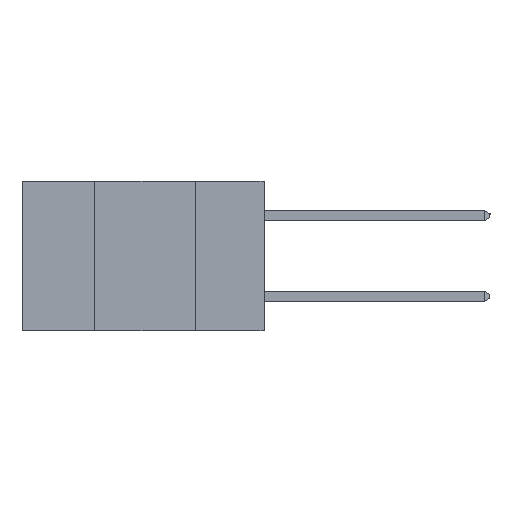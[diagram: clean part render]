
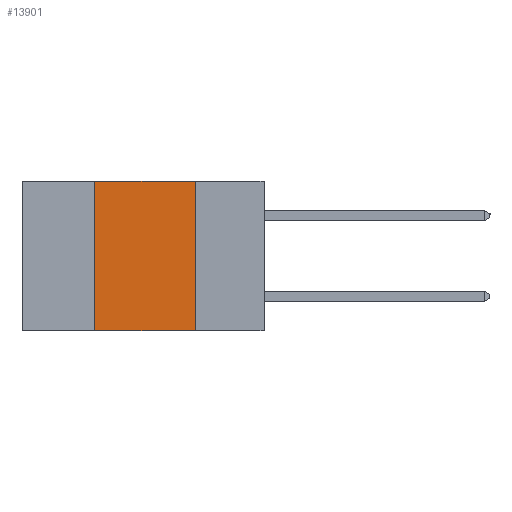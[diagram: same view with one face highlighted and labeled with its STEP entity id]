
A CAD part, left-side view. The second image highlights one B-rep face of the part: STEP entity #13901.
In plain terms, the highlighted planar face has unit normal (-1, 0, 0).
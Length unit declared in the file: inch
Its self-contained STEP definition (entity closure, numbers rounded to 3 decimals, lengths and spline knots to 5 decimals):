
#618 = EDGE_CURVE ( 'NONE', #12036, #2207, #12353, .T. ) ;
#1179 = CARTESIAN_POINT ( 'NONE',  ( 0., 0.6, 0. ) ) ;
#1736 = ORIENTED_EDGE ( 'NONE', *, *, #618, .F. ) ;
#1987 = DIRECTION ( 'NONE',  ( 0., 0., -1. ) ) ;
#2114 = ORIENTED_EDGE ( 'NONE', *, *, #3849, .F. ) ;
#2206 = DIRECTION ( 'NONE',  ( 0., -1., 0. ) ) ;
#2207 = VERTEX_POINT ( 'NONE', #3233 ) ;
#3233 = CARTESIAN_POINT ( 'NONE',  ( 0., 0.17, 0. ) ) ;
#3514 = AXIS2_PLACEMENT_3D ( 'NONE', #7386, #8438, #1987 ) ;
#3680 = VECTOR ( 'NONE', #2206, 39.37008 ) ;
#3693 = ORIENTED_EDGE ( 'NONE', *, *, #11956, .F. ) ;
#3723 = CARTESIAN_POINT ( 'NONE',  ( 0., 0.17, 0. ) ) ;
#3849 = EDGE_CURVE ( 'NONE', #11687, #12036, #4793, .T. ) ;
#4117 = VECTOR ( 'NONE', #4832, 39.37008 ) ;
#4793 = LINE ( 'NONE', #12039, #7367 ) ;
#4832 = DIRECTION ( 'NONE',  ( 0., 0., -1. ) ) ;
#6287 = PLANE ( 'NONE',  #3514 ) ;
#6577 = CARTESIAN_POINT ( 'NONE',  ( 0., 0.42, -0.37 ) ) ;
#6735 = CARTESIAN_POINT ( 'NONE',  ( 0., 0.6, -0.37 ) ) ;
#6781 = DIRECTION ( 'NONE',  ( 0., -1., 0. ) ) ;
#6821 = FACE_OUTER_BOUND ( 'NONE', #9806, .T. ) ;
#7367 = VECTOR ( 'NONE', #11407, 39.37008 ) ;
#7386 = CARTESIAN_POINT ( 'NONE',  ( 0., 0.6, 0. ) ) ;
#8438 = DIRECTION ( 'NONE',  ( 1., 0., 0. ) ) ;
#8745 = LINE ( 'NONE', #6735, #11304 ) ;
#9363 = EDGE_CURVE ( 'NONE', #11687, #9488, #8745, .T. ) ;
#9488 = VERTEX_POINT ( 'NONE', #11767 ) ;
#9806 = EDGE_LOOP ( 'NONE', ( #3693, #1736, #2114, #13989 ) ) ;
#11304 = VECTOR ( 'NONE', #6781, 39.37008 ) ;
#11407 = DIRECTION ( 'NONE',  ( 0., 0., 1. ) ) ;
#11687 = VERTEX_POINT ( 'NONE', #6577 ) ;
#11767 = CARTESIAN_POINT ( 'NONE',  ( 0., 0.17, -0.37 ) ) ;
#11956 = EDGE_CURVE ( 'NONE', #2207, #9488, #13119, .T. ) ;
#12036 = VERTEX_POINT ( 'NONE', #13609 ) ;
#12039 = CARTESIAN_POINT ( 'NONE',  ( 0., 0.42, 0. ) ) ;
#12353 = LINE ( 'NONE', #1179, #3680 ) ;
#13119 = LINE ( 'NONE', #3723, #4117 ) ;
#13609 = CARTESIAN_POINT ( 'NONE',  ( 0., 0.42, 0. ) ) ;
#13901 = ADVANCED_FACE ( 'NONE', ( #6821 ), #6287, .F. ) ;
#13989 = ORIENTED_EDGE ( 'NONE', *, *, #9363, .T. ) ;
